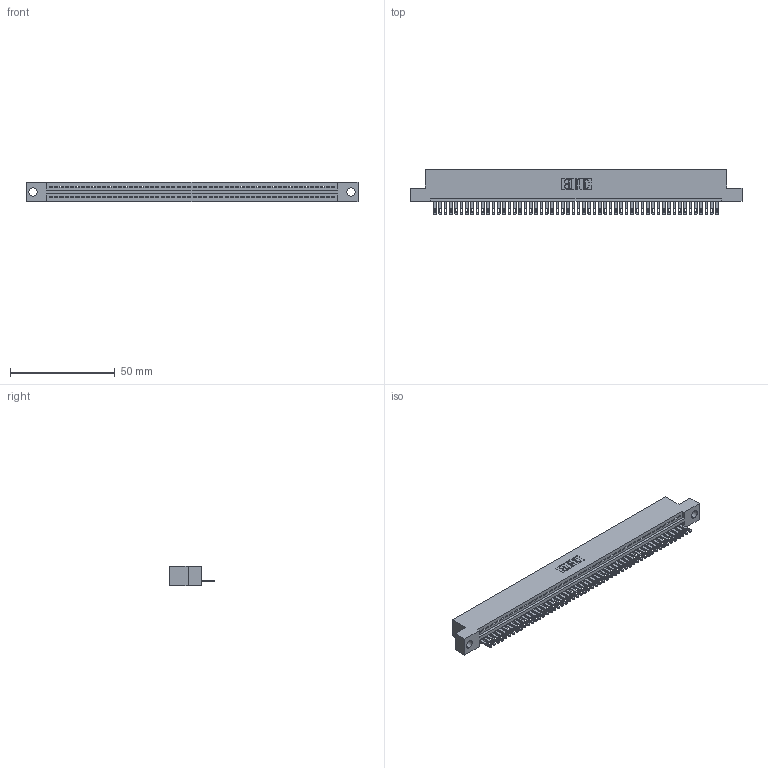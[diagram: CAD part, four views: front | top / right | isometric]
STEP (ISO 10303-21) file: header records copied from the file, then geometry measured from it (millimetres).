
FILE_DESCRIPTION (( 'STEP AP203' ), '1' );
FILE_NAME ('345-054-500-104.STEP', '2018-09-23T19:37:49', ( '' ), ( '' ), 'SwSTEP 2.0', 'SolidWorks 2016', '' );
FILE_SCHEMA (( 'CONFIG_CONTROL_DESIGN' ));
Length unit declared in the file: inch
Products named in the file (3): 345 Part_Flush Mounting Lugs - 0.156 Dia-TH; 345-292-001_345-293-100; 345-054-500-104
Assembly tree (55 placements, depth 2):
  345-054-500-104
    345 Part_Flush Mounting Lugs - 0.156 Dia-TH
    345-292-001_345-293-100  x54
Bounding box: 158.37 x 21.51 x 9.4 mm (x, y, z)
Volume: 15085.9 mm3; surface area: 20140.9 mm2
Topology: 55 solids, 55 shells, 3042 faces, 9413 edges, 6274 vertices
Faces by surface type: plane 1916, cylinder 1126
Entity records: 38959 total; most frequent: CARTESIAN_POINT 6754, ORIENTED_EDGE 6742, DIRECTION 5883, EDGE_CURVE 3371, VECTOR 3019, LINE 3019, VERTEX_POINT 2246, AXIS2_PLACEMENT_3D 1432
